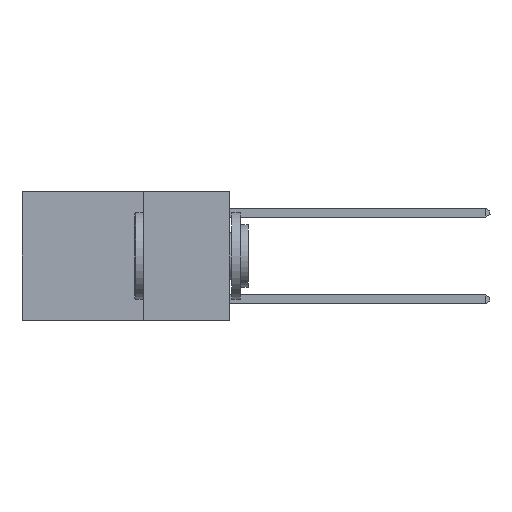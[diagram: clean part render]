
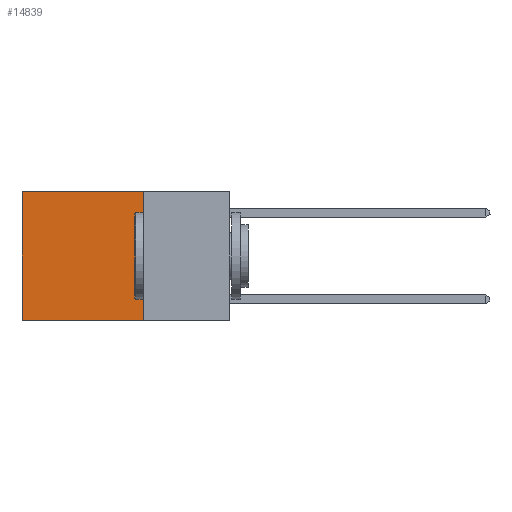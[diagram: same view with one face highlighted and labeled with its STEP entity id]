
A CAD part, left-side view. The second image highlights one B-rep face of the part: STEP entity #14839.
In plain terms, the highlighted planar face has unit normal (-1, 0, 0).
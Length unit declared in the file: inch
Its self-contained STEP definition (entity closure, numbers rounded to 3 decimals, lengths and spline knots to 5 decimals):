
#23 = CARTESIAN_POINT ( 'NONE',  ( 0.2625, 0.25, -0.37 ) ) ;
#232 = LINE ( 'NONE', #4478, #4312 ) ;
#1202 = DIRECTION ( 'NONE',  ( 0., 0., -1. ) ) ;
#1711 = VECTOR ( 'NONE', #2757, 39.37008 ) ;
#1734 = ORIENTED_EDGE ( 'NONE', *, *, #15816, .F. ) ;
#1883 = EDGE_LOOP ( 'NONE', ( #14282, #6750, #1734, #14011 ) ) ;
#2411 = VECTOR ( 'NONE', #6144, 39.37008 ) ;
#2757 = DIRECTION ( 'NONE',  ( 0., 0., -1. ) ) ;
#3503 = CARTESIAN_POINT ( 'NONE',  ( 0.2625, 0.25, 0. ) ) ;
#4137 = VECTOR ( 'NONE', #1202, 39.37008 ) ;
#4200 = CARTESIAN_POINT ( 'NONE',  ( 0.2625, 0.25, 0. ) ) ;
#4312 = VECTOR ( 'NONE', #12680, 39.37008 ) ;
#4478 = CARTESIAN_POINT ( 'NONE',  ( 0.2625, 0.25, -0.37 ) ) ;
#4517 = EDGE_CURVE ( 'NONE', #14483, #12956, #10891, .T. ) ;
#4608 = CARTESIAN_POINT ( 'NONE',  ( 0.2625, 0.6, -0.37 ) ) ;
#5094 = LINE ( 'NONE', #7918, #4137 ) ;
#6144 = DIRECTION ( 'NONE',  ( 0., 1., 0. ) ) ;
#6750 = ORIENTED_EDGE ( 'NONE', *, *, #10261, .F. ) ;
#7918 = CARTESIAN_POINT ( 'NONE',  ( 0.2625, 0.25, 0. ) ) ;
#8931 = DIRECTION ( 'NONE',  ( 1., 0., 0. ) ) ;
#9526 = CARTESIAN_POINT ( 'NONE',  ( 0.2625, 0.6, 0. ) ) ;
#10261 = EDGE_CURVE ( 'NONE', #17397, #12956, #232, .T. ) ;
#10891 = LINE ( 'NONE', #9526, #1711 ) ;
#11352 = LINE ( 'NONE', #11434, #2411 ) ;
#11434 = CARTESIAN_POINT ( 'NONE',  ( 0.2625, 0.25, 0. ) ) ;
#12343 = VERTEX_POINT ( 'NONE', #4200 ) ;
#12644 = AXIS2_PLACEMENT_3D ( 'NONE', #3503, #8931, #17028 ) ;
#12680 = DIRECTION ( 'NONE',  ( 0., 1., 0. ) ) ;
#12956 = VERTEX_POINT ( 'NONE', #4608 ) ;
#13990 = EDGE_CURVE ( 'NONE', #12343, #14483, #11352, .T. ) ;
#14011 = ORIENTED_EDGE ( 'NONE', *, *, #13990, .T. ) ;
#14214 = FACE_OUTER_BOUND ( 'NONE', #1883, .T. ) ;
#14235 = CARTESIAN_POINT ( 'NONE',  ( 0.2625, 0.6, 0. ) ) ;
#14282 = ORIENTED_EDGE ( 'NONE', *, *, #4517, .T. ) ;
#14483 = VERTEX_POINT ( 'NONE', #14235 ) ;
#14839 = ADVANCED_FACE ( 'NONE', ( #14214 ), #17201, .F. ) ;
#15816 = EDGE_CURVE ( 'NONE', #12343, #17397, #5094, .T. ) ;
#17028 = DIRECTION ( 'NONE',  ( 0., 0., -1. ) ) ;
#17201 = PLANE ( 'NONE',  #12644 ) ;
#17397 = VERTEX_POINT ( 'NONE', #23 ) ;
